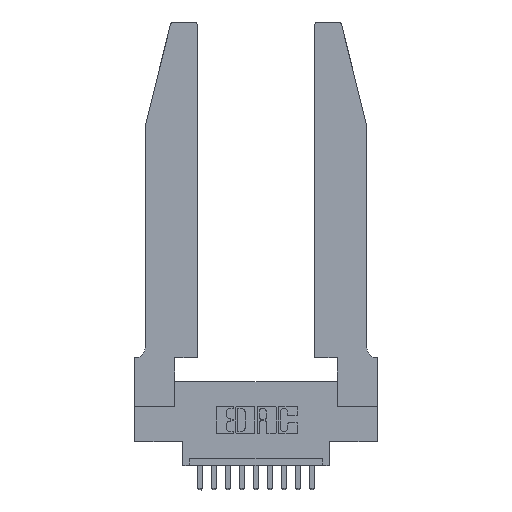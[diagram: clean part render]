
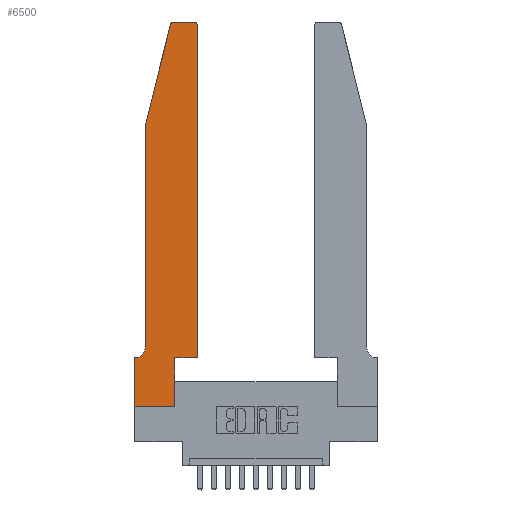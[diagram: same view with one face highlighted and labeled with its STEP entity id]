
A CAD part, top view. The second image highlights one B-rep face of the part: STEP entity #6500.
In plain terms, the highlighted planar face has unit normal (0, 0, 1).
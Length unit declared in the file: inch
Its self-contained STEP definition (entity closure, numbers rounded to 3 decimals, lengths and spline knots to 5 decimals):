
#507 = VERTEX_POINT ( 'NONE', #12628 ) ;
#651 = CARTESIAN_POINT ( 'NONE',  ( 0.25487, 2.72718, 0.37 ) ) ;
#891 = CARTESIAN_POINT ( 'NONE',  ( 0.0755, 2., 0.37 ) ) ;
#1340 = CARTESIAN_POINT ( 'NONE',  ( 0.0755, 2., 0.37 ) ) ;
#1550 = LINE ( 'NONE', #15448, #11762 ) ;
#1706 = DIRECTION ( 'NONE',  ( 0., 0., 1. ) ) ;
#2000 = AXIS2_PLACEMENT_3D ( 'NONE', #7539, #6127, #2420 ) ;
#2260 = ORIENTED_EDGE ( 'NONE', *, *, #4803, .T. ) ;
#2420 = DIRECTION ( 'NONE',  ( 1., 0., 0. ) ) ;
#2642 = DIRECTION ( 'NONE',  ( -0.239, -0.971, 0. ) ) ;
#3041 = CARTESIAN_POINT ( 'NONE',  ( 0.0755, 0.42, 0.37 ) ) ;
#3046 = ORIENTED_EDGE ( 'NONE', *, *, #14386, .T. ) ;
#3122 = EDGE_CURVE ( 'NONE', #15804, #4281, #13066, .T. ) ;
#3602 = FACE_OUTER_BOUND ( 'NONE', #5147, .T. ) ;
#3860 = ORIENTED_EDGE ( 'NONE', *, *, #11488, .T. ) ;
#4028 = ORIENTED_EDGE ( 'NONE', *, *, #3122, .T. ) ;
#4055 = VERTEX_POINT ( 'NONE', #10126 ) ;
#4209 = VECTOR ( 'NONE', #7492, 39.37008 ) ;
#4281 = VERTEX_POINT ( 'NONE', #12139 ) ;
#4803 = EDGE_CURVE ( 'NONE', #5962, #5908, #15962, .T. ) ;
#4854 = CARTESIAN_POINT ( 'NONE',  ( 0.284, 2.75, 0.37 ) ) ;
#4914 = ORIENTED_EDGE ( 'NONE', *, *, #11940, .T. ) ;
#5147 = EDGE_LOOP ( 'NONE', ( #9673, #8945, #4914, #5809, #11697, #2260, #3046, #6862, #15298, #9996, #3860, #4028 ) ) ;
#5253 = LINE ( 'NONE', #891, #5636 ) ;
#5270 = VECTOR ( 'NONE', #2642, 39.37008 ) ;
#5557 = CARTESIAN_POINT ( 'NONE',  ( 0., 0., 0.37 ) ) ;
#5636 = VECTOR ( 'NONE', #12406, 39.37008 ) ;
#5750 = VECTOR ( 'NONE', #6354, 39.37008 ) ;
#5762 = EDGE_CURVE ( 'NONE', #11317, #5962, #7694, .T. ) ;
#5809 = ORIENTED_EDGE ( 'NONE', *, *, #12197, .T. ) ;
#5904 = CARTESIAN_POINT ( 'NONE',  ( 0.0055, 0.35, 0.37 ) ) ;
#5908 = VERTEX_POINT ( 'NONE', #13881 ) ;
#5934 = EDGE_CURVE ( 'NONE', #4281, #15327, #7900, .T. ) ;
#5962 = VERTEX_POINT ( 'NONE', #5904 ) ;
#6127 = DIRECTION ( 'NONE',  ( 0., 0., 1. ) ) ;
#6354 = DIRECTION ( 'NONE',  ( -1., 0., 0. ) ) ;
#6500 = ADVANCED_FACE ( 'NONE', ( #3602 ), #6981, .T. ) ;
#6726 = CARTESIAN_POINT ( 'NONE',  ( 0.2865, 0., 0.37 ) ) ;
#6777 = AXIS2_PLACEMENT_3D ( 'NONE', #8143, #15751, #15802 ) ;
#6862 = ORIENTED_EDGE ( 'NONE', *, *, #13943, .T. ) ;
#6981 = PLANE ( 'NONE',  #12949 ) ;
#7077 = CARTESIAN_POINT ( 'NONE',  ( 0.0755, 2., 0.37 ) ) ;
#7152 = VECTOR ( 'NONE', #9518, 39.37008 ) ;
#7215 = VERTEX_POINT ( 'NONE', #6726 ) ;
#7253 = DIRECTION ( 'NONE',  ( 0., 1., 0. ) ) ;
#7366 = CARTESIAN_POINT ( 'NONE',  ( 0.2865, 0.35, 0.37 ) ) ;
#7492 = DIRECTION ( 'NONE',  ( -1., 0., 0. ) ) ;
#7539 = CARTESIAN_POINT ( 'NONE',  ( 0.4205, 2.72, 0.37 ) ) ;
#7694 = CIRCLE ( 'NONE', #6777, 0.07 ) ;
#7900 = LINE ( 'NONE', #13634, #5750 ) ;
#8094 = VECTOR ( 'NONE', #7253, 39.37008 ) ;
#8143 = CARTESIAN_POINT ( 'NONE',  ( 0.0055, 0.42, 0.37 ) ) ;
#8169 = DIRECTION ( 'NONE',  ( 0., 0., 1. ) ) ;
#8395 = EDGE_CURVE ( 'NONE', #7215, #4055, #10265, .T. ) ;
#8945 = ORIENTED_EDGE ( 'NONE', *, *, #11466, .T. ) ;
#9518 = DIRECTION ( 'NONE',  ( 1., 0., 0. ) ) ;
#9541 = DIRECTION ( 'NONE',  ( 1., 0., 0. ) ) ;
#9673 = ORIENTED_EDGE ( 'NONE', *, *, #5934, .T. ) ;
#9996 = ORIENTED_EDGE ( 'NONE', *, *, #14585, .T. ) ;
#10126 = CARTESIAN_POINT ( 'NONE',  ( 0.2865, 0.35, 0.37 ) ) ;
#10265 = LINE ( 'NONE', #7366, #8094 ) ;
#10606 = CARTESIAN_POINT ( 'NONE',  ( 0., 0., 0.37 ) ) ;
#10684 = LINE ( 'NONE', #12766, #11092 ) ;
#10748 = VERTEX_POINT ( 'NONE', #5557 ) ;
#10869 = CARTESIAN_POINT ( 'NONE',  ( 0., 0.35, 0.37 ) ) ;
#11092 = VECTOR ( 'NONE', #11580, 39.37008 ) ;
#11317 = VERTEX_POINT ( 'NONE', #3041 ) ;
#11466 = EDGE_CURVE ( 'NONE', #15327, #12660, #14477, .T. ) ;
#11488 = EDGE_CURVE ( 'NONE', #507, #15804, #1550, .T. ) ;
#11580 = DIRECTION ( 'NONE',  ( 0., -1., 0. ) ) ;
#11697 = ORIENTED_EDGE ( 'NONE', *, *, #5762, .T. ) ;
#11701 = CARTESIAN_POINT ( 'NONE',  ( 0.284, 2.72, 0.37 ) ) ;
#11762 = VECTOR ( 'NONE', #14193, 39.37008 ) ;
#11940 = EDGE_CURVE ( 'NONE', #12660, #12733, #14648, .T. ) ;
#12139 = CARTESIAN_POINT ( 'NONE',  ( 0.4205, 2.75, 0.37 ) ) ;
#12197 = EDGE_CURVE ( 'NONE', #12733, #11317, #5253, .T. ) ;
#12406 = DIRECTION ( 'NONE',  ( 0., -1., 0. ) ) ;
#12628 = CARTESIAN_POINT ( 'NONE',  ( 0.4505, 0.35, 0.37 ) ) ;
#12645 = VECTOR ( 'NONE', #15549, 39.37008 ) ;
#12660 = VERTEX_POINT ( 'NONE', #651 ) ;
#12733 = VERTEX_POINT ( 'NONE', #7077 ) ;
#12766 = CARTESIAN_POINT ( 'NONE',  ( 0., 0., 0.37 ) ) ;
#12934 = DIRECTION ( 'NONE',  ( 1., 0., 0. ) ) ;
#12949 = AXIS2_PLACEMENT_3D ( 'NONE', #10869, #8169, #9541 ) ;
#13066 = CIRCLE ( 'NONE', #2000, 0.03 ) ;
#13145 = CARTESIAN_POINT ( 'NONE',  ( 0.4505, 2.72, 0.37 ) ) ;
#13634 = CARTESIAN_POINT ( 'NONE',  ( 0.2605, 2.75, 0.37 ) ) ;
#13803 = LINE ( 'NONE', #15428, #7152 ) ;
#13881 = CARTESIAN_POINT ( 'NONE',  ( 0., 0.35, 0.37 ) ) ;
#13943 = EDGE_CURVE ( 'NONE', #10748, #7215, #15969, .T. ) ;
#14193 = DIRECTION ( 'NONE',  ( 0., 1., 0. ) ) ;
#14354 = AXIS2_PLACEMENT_3D ( 'NONE', #11701, #1706, #12934 ) ;
#14386 = EDGE_CURVE ( 'NONE', #5908, #10748, #10684, .T. ) ;
#14477 = CIRCLE ( 'NONE', #14354, 0.03 ) ;
#14585 = EDGE_CURVE ( 'NONE', #4055, #507, #13803, .T. ) ;
#14648 = LINE ( 'NONE', #1340, #5270 ) ;
#14960 = CARTESIAN_POINT ( 'NONE',  ( 0.0755, 0.35, 0.37 ) ) ;
#15298 = ORIENTED_EDGE ( 'NONE', *, *, #8395, .T. ) ;
#15327 = VERTEX_POINT ( 'NONE', #4854 ) ;
#15428 = CARTESIAN_POINT ( 'NONE',  ( 0.4505, 0.35, 0.37 ) ) ;
#15448 = CARTESIAN_POINT ( 'NONE',  ( 0.4505, 0.35, 0.37 ) ) ;
#15549 = DIRECTION ( 'NONE',  ( 1., 0., 0. ) ) ;
#15751 = DIRECTION ( 'NONE',  ( 0., 0., -1. ) ) ;
#15802 = DIRECTION ( 'NONE',  ( -1., 0., 0. ) ) ;
#15804 = VERTEX_POINT ( 'NONE', #13145 ) ;
#15962 = LINE ( 'NONE', #14960, #4209 ) ;
#15969 = LINE ( 'NONE', #10606, #12645 ) ;
